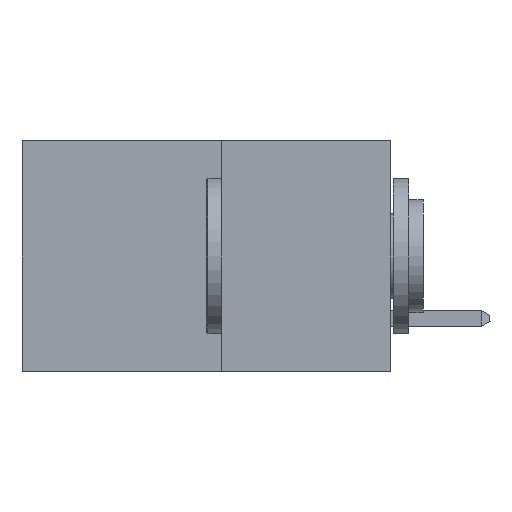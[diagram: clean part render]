
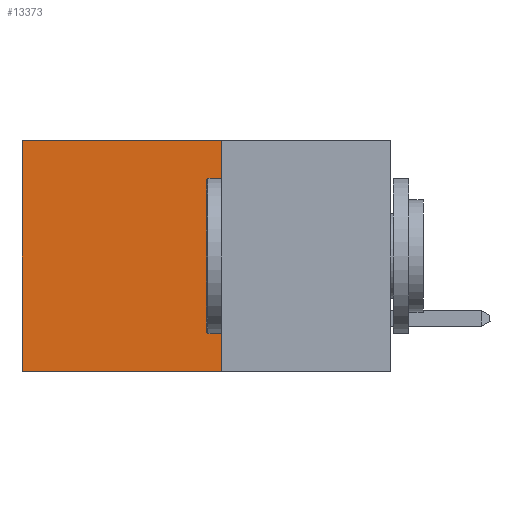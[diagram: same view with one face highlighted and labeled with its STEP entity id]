
A CAD part, left-side view. The second image highlights one B-rep face of the part: STEP entity #13373.
In plain terms, the highlighted planar face has unit normal (-1, 0, 0).
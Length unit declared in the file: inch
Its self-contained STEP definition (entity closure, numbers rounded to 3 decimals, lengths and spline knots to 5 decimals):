
#238 = LINE ( 'NONE', #9063, #6250 ) ;
#353 = LINE ( 'NONE', #20213, #26647 ) ;
#2683 = ORIENTED_EDGE ( 'NONE', *, *, #7506, .F. ) ;
#3045 = CARTESIAN_POINT ( 'NONE',  ( 0.277, 0.59, 0. ) ) ;
#3445 = CARTESIAN_POINT ( 'NONE',  ( 0.277, 0.59, -0.37 ) ) ;
#5889 = ORIENTED_EDGE ( 'NONE', *, *, #24228, .T. ) ;
#5972 = VECTOR ( 'NONE', #6267, 39.37008 ) ;
#6250 = VECTOR ( 'NONE', #11619, 39.37008 ) ;
#6267 = DIRECTION ( 'NONE',  ( 0., 1., 0. ) ) ;
#6389 = CARTESIAN_POINT ( 'NONE',  ( 0.277, 0.27, -0.37 ) ) ;
#7506 = EDGE_CURVE ( 'NONE', #32638, #23176, #27067, .T. ) ;
#8398 = EDGE_CURVE ( 'NONE', #9555, #32638, #353, .T. ) ;
#9063 = CARTESIAN_POINT ( 'NONE',  ( 0.277, 0.59, -0.37 ) ) ;
#9555 = VERTEX_POINT ( 'NONE', #29611 ) ;
#10543 = DIRECTION ( 'NONE',  ( 0., 0., -1. ) ) ;
#10557 = EDGE_LOOP ( 'NONE', ( #21578, #2683, #29766, #5889 ) ) ;
#11016 = CARTESIAN_POINT ( 'NONE',  ( 0.277, 0.27, -0.37 ) ) ;
#11619 = DIRECTION ( 'NONE',  ( 0., 0., -1. ) ) ;
#12253 = AXIS2_PLACEMENT_3D ( 'NONE', #23185, #25710, #10543 ) ;
#13373 = ADVANCED_FACE ( 'NONE', ( #28699 ), #20638, .F. ) ;
#14808 = LINE ( 'NONE', #17673, #26770 ) ;
#17673 = CARTESIAN_POINT ( 'NONE',  ( 0.277, 0.27, 0. ) ) ;
#20213 = CARTESIAN_POINT ( 'NONE',  ( 0.277, 0.27, -0.37 ) ) ;
#20272 = DIRECTION ( 'NONE',  ( 0., 1., 0. ) ) ;
#20638 = PLANE ( 'NONE',  #12253 ) ;
#21578 = ORIENTED_EDGE ( 'NONE', *, *, #21884, .T. ) ;
#21884 = EDGE_CURVE ( 'NONE', #22300, #23176, #238, .T. ) ;
#22300 = VERTEX_POINT ( 'NONE', #3045 ) ;
#23176 = VERTEX_POINT ( 'NONE', #3445 ) ;
#23185 = CARTESIAN_POINT ( 'NONE',  ( 0.277, 0.27, -0.37 ) ) ;
#24228 = EDGE_CURVE ( 'NONE', #9555, #22300, #14808, .T. ) ;
#25297 = DIRECTION ( 'NONE',  ( 0., 0., -1. ) ) ;
#25710 = DIRECTION ( 'NONE',  ( 1., 0., 0. ) ) ;
#26647 = VECTOR ( 'NONE', #25297, 39.37008 ) ;
#26770 = VECTOR ( 'NONE', #20272, 39.37008 ) ;
#27067 = LINE ( 'NONE', #6389, #5972 ) ;
#28699 = FACE_OUTER_BOUND ( 'NONE', #10557, .T. ) ;
#29611 = CARTESIAN_POINT ( 'NONE',  ( 0.277, 0.27, 0. ) ) ;
#29766 = ORIENTED_EDGE ( 'NONE', *, *, #8398, .F. ) ;
#32638 = VERTEX_POINT ( 'NONE', #11016 ) ;
